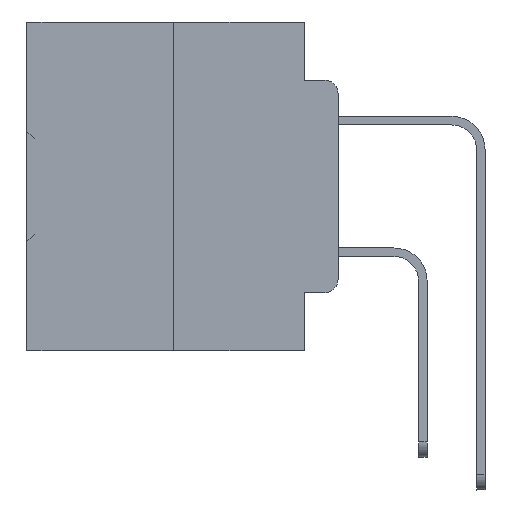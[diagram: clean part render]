
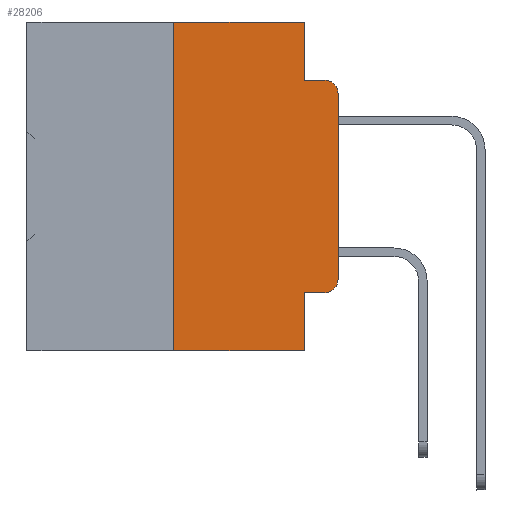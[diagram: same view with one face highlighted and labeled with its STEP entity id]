
A CAD part, left-side view. The second image highlights one B-rep face of the part: STEP entity #28206.
In plain terms, the highlighted planar face has unit normal (-1, 0, 0).
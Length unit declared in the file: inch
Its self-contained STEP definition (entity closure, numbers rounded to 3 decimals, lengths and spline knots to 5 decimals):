
#244 = EDGE_LOOP ( 'NONE', ( #7874, #33793, #7710, #11575, #13857, #12124, #8412, #27384, #9655, #17254 ) ) ;
#325 = CARTESIAN_POINT ( 'NONE',  ( 0., 0.02, -0.0885 ) ) ;
#1354 = VERTEX_POINT ( 'NONE', #36675 ) ;
#1686 = DIRECTION ( 'NONE',  ( 0., -1., 0. ) ) ;
#1948 = DIRECTION ( 'NONE',  ( 0., -1., 0. ) ) ;
#2472 = VERTEX_POINT ( 'NONE', #6852 ) ;
#3156 = DIRECTION ( 'NONE',  ( 0., 0., -1. ) ) ;
#3980 = VERTEX_POINT ( 'NONE', #15076 ) ;
#5763 = LINE ( 'NONE', #38603, #13322 ) ;
#5858 = VECTOR ( 'NONE', #12834, 39.37008 ) ;
#6852 = CARTESIAN_POINT ( 'NONE',  ( 0., 0.051, -0.4115 ) ) ;
#7091 = VECTOR ( 'NONE', #1948, 39.37008 ) ;
#7710 = ORIENTED_EDGE ( 'NONE', *, *, #16587, .F. ) ;
#7874 = ORIENTED_EDGE ( 'NONE', *, *, #36195, .T. ) ;
#8412 = ORIENTED_EDGE ( 'NONE', *, *, #40842, .T. ) ;
#9655 = ORIENTED_EDGE ( 'NONE', *, *, #28256, .T. ) ;
#9904 = CARTESIAN_POINT ( 'NONE',  ( 0., 0., -0.1085 ) ) ;
#10654 = DIRECTION ( 'NONE',  ( 0., 0., 1. ) ) ;
#11462 = CARTESIAN_POINT ( 'NONE',  ( 0., 0.25, 0. ) ) ;
#11575 = ORIENTED_EDGE ( 'NONE', *, *, #17998, .F. ) ;
#12124 = ORIENTED_EDGE ( 'NONE', *, *, #40248, .F. ) ;
#12834 = DIRECTION ( 'NONE',  ( 0., 0., -1. ) ) ;
#13322 = VECTOR ( 'NONE', #29248, 39.37008 ) ;
#13339 = PLANE ( 'NONE',  #16199 ) ;
#13729 = VERTEX_POINT ( 'NONE', #21707 ) ;
#13857 = ORIENTED_EDGE ( 'NONE', *, *, #23287, .F. ) ;
#14241 = DIRECTION ( 'NONE',  ( -1., 0., 0. ) ) ;
#14333 = LINE ( 'NONE', #11462, #21768 ) ;
#14939 = VERTEX_POINT ( 'NONE', #32548 ) ;
#15076 = CARTESIAN_POINT ( 'NONE',  ( 0., 0., -0.3915 ) ) ;
#15196 = LINE ( 'NONE', #33466, #38275 ) ;
#15713 = DIRECTION ( 'NONE',  ( 0., -1., 0. ) ) ;
#15749 = VERTEX_POINT ( 'NONE', #23775 ) ;
#16199 = AXIS2_PLACEMENT_3D ( 'NONE', #35301, #38467, #19716 ) ;
#16587 = EDGE_CURVE ( 'NONE', #1354, #39952, #25089, .T. ) ;
#17254 = ORIENTED_EDGE ( 'NONE', *, *, #23150, .T. ) ;
#17998 = EDGE_CURVE ( 'NONE', #24062, #1354, #15196, .T. ) ;
#18523 = VERTEX_POINT ( 'NONE', #23885 ) ;
#19448 = EDGE_CURVE ( 'NONE', #22318, #39952, #19563, .T. ) ;
#19563 = CIRCLE ( 'NONE', #33907, 0.02 ) ;
#19716 = DIRECTION ( 'NONE',  ( 0., 0., -1. ) ) ;
#21707 = CARTESIAN_POINT ( 'NONE',  ( 0., 0.02, -0.4115 ) ) ;
#21768 = VECTOR ( 'NONE', #39705, 39.37008 ) ;
#22313 = DIRECTION ( 'NONE',  ( -1., 0., 0. ) ) ;
#22318 = VERTEX_POINT ( 'NONE', #9904 ) ;
#22575 = CIRCLE ( 'NONE', #27946, 0.02 ) ;
#23150 = EDGE_CURVE ( 'NONE', #13729, #3980, #22575, .T. ) ;
#23287 = EDGE_CURVE ( 'NONE', #15749, #24062, #24978, .T. ) ;
#23775 = CARTESIAN_POINT ( 'NONE',  ( 0., 0.25, 0. ) ) ;
#23885 = CARTESIAN_POINT ( 'NONE',  ( 0., 0.051, -0.5 ) ) ;
#24035 = DIRECTION ( 'NONE',  ( 0., 0., -1. ) ) ;
#24062 = VERTEX_POINT ( 'NONE', #32264 ) ;
#24129 = VECTOR ( 'NONE', #15713, 39.37008 ) ;
#24659 = FACE_OUTER_BOUND ( 'NONE', #244, .T. ) ;
#24978 = LINE ( 'NONE', #39919, #7091 ) ;
#25089 = LINE ( 'NONE', #31332, #24129 ) ;
#25100 = LINE ( 'NONE', #39661, #32431 ) ;
#27384 = ORIENTED_EDGE ( 'NONE', *, *, #33209, .F. ) ;
#27946 = AXIS2_PLACEMENT_3D ( 'NONE', #33052, #14241, #36210 ) ;
#28206 = ADVANCED_FACE ( 'NONE', ( #24659 ), #13339, .F. ) ;
#28256 = EDGE_CURVE ( 'NONE', #2472, #13729, #5763, .T. ) ;
#28947 = VECTOR ( 'NONE', #10654, 39.37008 ) ;
#29248 = DIRECTION ( 'NONE',  ( 0., -1., 0. ) ) ;
#31096 = LINE ( 'NONE', #31648, #5858 ) ;
#31332 = CARTESIAN_POINT ( 'NONE',  ( 0., 0.051, -0.0885 ) ) ;
#31648 = CARTESIAN_POINT ( 'NONE',  ( 0., 0.051, 0. ) ) ;
#32264 = CARTESIAN_POINT ( 'NONE',  ( 0., 0.051, 0. ) ) ;
#32431 = VECTOR ( 'NONE', #1686, 39.37008 ) ;
#32548 = CARTESIAN_POINT ( 'NONE',  ( 0., 0.25, -0.5 ) ) ;
#32726 = CARTESIAN_POINT ( 'NONE',  ( 0., 0., 0. ) ) ;
#33052 = CARTESIAN_POINT ( 'NONE',  ( 0., 0.02, -0.3915 ) ) ;
#33209 = EDGE_CURVE ( 'NONE', #2472, #18523, #31096, .T. ) ;
#33466 = CARTESIAN_POINT ( 'NONE',  ( 0., 0.051, 0. ) ) ;
#33793 = ORIENTED_EDGE ( 'NONE', *, *, #19448, .T. ) ;
#33907 = AXIS2_PLACEMENT_3D ( 'NONE', #41067, #22313, #3156 ) ;
#35301 = CARTESIAN_POINT ( 'NONE',  ( 0., 0.473, 0. ) ) ;
#36195 = EDGE_CURVE ( 'NONE', #3980, #22318, #37300, .T. ) ;
#36210 = DIRECTION ( 'NONE',  ( 0., 0., -1. ) ) ;
#36675 = CARTESIAN_POINT ( 'NONE',  ( 0., 0.051, -0.0885 ) ) ;
#37300 = LINE ( 'NONE', #32726, #28947 ) ;
#38275 = VECTOR ( 'NONE', #24035, 39.37008 ) ;
#38467 = DIRECTION ( 'NONE',  ( 1., 0., 0. ) ) ;
#38603 = CARTESIAN_POINT ( 'NONE',  ( 0., 0.051, -0.4115 ) ) ;
#39661 = CARTESIAN_POINT ( 'NONE',  ( 0., 0.473, -0.5 ) ) ;
#39705 = DIRECTION ( 'NONE',  ( 0., 0., 1. ) ) ;
#39919 = CARTESIAN_POINT ( 'NONE',  ( 0., 0.473, 0. ) ) ;
#39952 = VERTEX_POINT ( 'NONE', #325 ) ;
#40248 = EDGE_CURVE ( 'NONE', #14939, #15749, #14333, .T. ) ;
#40842 = EDGE_CURVE ( 'NONE', #14939, #18523, #25100, .T. ) ;
#41067 = CARTESIAN_POINT ( 'NONE',  ( 0., 0.02, -0.1085 ) ) ;
